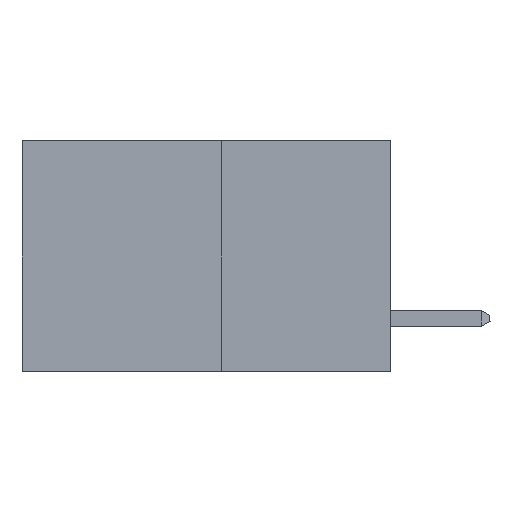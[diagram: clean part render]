
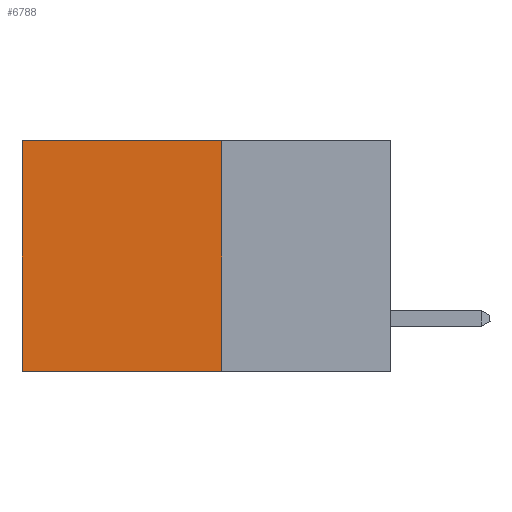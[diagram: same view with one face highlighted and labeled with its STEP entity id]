
A CAD part, left-side view. The second image highlights one B-rep face of the part: STEP entity #6788.
In plain terms, the highlighted planar face has unit normal (-1, 0, 0).
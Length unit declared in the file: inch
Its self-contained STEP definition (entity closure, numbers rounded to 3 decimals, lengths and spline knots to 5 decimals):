
#172 = VERTEX_POINT ( 'NONE', #10796 ) ;
#601 = CARTESIAN_POINT ( 'NONE',  ( 0.277, 0.27, -0.37 ) ) ;
#699 = CARTESIAN_POINT ( 'NONE',  ( 0.277, 0.59, -0.37 ) ) ;
#1228 = VERTEX_POINT ( 'NONE', #17224 ) ;
#1745 = CARTESIAN_POINT ( 'NONE',  ( 0.277, 0.27, 0. ) ) ;
#1937 = EDGE_LOOP ( 'NONE', ( #1995, #5378, #8085, #12050 ) ) ;
#1995 = ORIENTED_EDGE ( 'NONE', *, *, #14534, .T. ) ;
#2101 = VERTEX_POINT ( 'NONE', #3074 ) ;
#2858 = LINE ( 'NONE', #8334, #10188 ) ;
#3074 = CARTESIAN_POINT ( 'NONE',  ( 0.277, 0.27, -0.37 ) ) ;
#5378 = ORIENTED_EDGE ( 'NONE', *, *, #12654, .F. ) ;
#5428 = VECTOR ( 'NONE', #11643, 39.37008 ) ;
#6663 = CARTESIAN_POINT ( 'NONE',  ( 0.277, 0.59, 0. ) ) ;
#6788 = ADVANCED_FACE ( 'NONE', ( #12961 ), #16628, .F. ) ;
#7045 = LINE ( 'NONE', #699, #13958 ) ;
#8085 = ORIENTED_EDGE ( 'NONE', *, *, #12427, .F. ) ;
#8334 = CARTESIAN_POINT ( 'NONE',  ( 0.277, 0.27, -0.37 ) ) ;
#9733 = DIRECTION ( 'NONE',  ( 0., 0., -1. ) ) ;
#10188 = VECTOR ( 'NONE', #9733, 39.37008 ) ;
#10279 = AXIS2_PLACEMENT_3D ( 'NONE', #16598, #16535, #16507 ) ;
#10796 = CARTESIAN_POINT ( 'NONE',  ( 0.277, 0.59, -0.37 ) ) ;
#11228 = EDGE_CURVE ( 'NONE', #1228, #11621, #11741, .T. ) ;
#11401 = DIRECTION ( 'NONE',  ( 0., 1., 0. ) ) ;
#11621 = VERTEX_POINT ( 'NONE', #6663 ) ;
#11643 = DIRECTION ( 'NONE',  ( 0., 1., 0. ) ) ;
#11741 = LINE ( 'NONE', #1745, #12163 ) ;
#12050 = ORIENTED_EDGE ( 'NONE', *, *, #11228, .T. ) ;
#12163 = VECTOR ( 'NONE', #11401, 39.37008 ) ;
#12427 = EDGE_CURVE ( 'NONE', #1228, #2101, #2858, .T. ) ;
#12654 = EDGE_CURVE ( 'NONE', #2101, #172, #12757, .T. ) ;
#12757 = LINE ( 'NONE', #601, #5428 ) ;
#12961 = FACE_OUTER_BOUND ( 'NONE', #1937, .T. ) ;
#13114 = DIRECTION ( 'NONE',  ( 0., 0., -1. ) ) ;
#13958 = VECTOR ( 'NONE', #13114, 39.37008 ) ;
#14534 = EDGE_CURVE ( 'NONE', #11621, #172, #7045, .T. ) ;
#16507 = DIRECTION ( 'NONE',  ( 0., 0., -1. ) ) ;
#16535 = DIRECTION ( 'NONE',  ( 1., 0., 0. ) ) ;
#16598 = CARTESIAN_POINT ( 'NONE',  ( 0.277, 0.27, -0.37 ) ) ;
#16628 = PLANE ( 'NONE',  #10279 ) ;
#17224 = CARTESIAN_POINT ( 'NONE',  ( 0.277, 0.27, 0. ) ) ;
